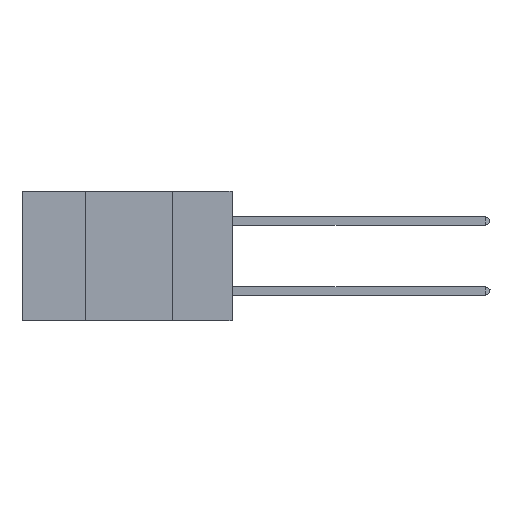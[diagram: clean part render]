
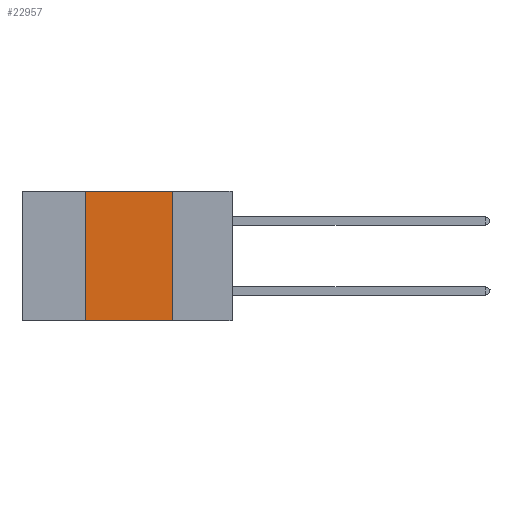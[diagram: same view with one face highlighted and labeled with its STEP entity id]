
A CAD part, left-side view. The second image highlights one B-rep face of the part: STEP entity #22957.
In plain terms, the highlighted planar face has unit normal (-1, 0, 0).
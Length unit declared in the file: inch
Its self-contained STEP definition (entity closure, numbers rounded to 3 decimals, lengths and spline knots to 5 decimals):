
#232 = LINE ( 'NONE', #357, #9091 ) ;
#357 = CARTESIAN_POINT ( 'NONE',  ( 0., 0.6, 0. ) ) ;
#1050 = FACE_OUTER_BOUND ( 'NONE', #24272, .T. ) ;
#2478 = CARTESIAN_POINT ( 'NONE',  ( 0., 0.17, 0. ) ) ;
#5051 = DIRECTION ( 'NONE',  ( 0., 0., 1. ) ) ;
#6407 = VERTEX_POINT ( 'NONE', #14930 ) ;
#6604 = CARTESIAN_POINT ( 'NONE',  ( 0., 0.6, -0.37 ) ) ;
#7446 = VECTOR ( 'NONE', #8625, 39.37008 ) ;
#7816 = EDGE_CURVE ( 'NONE', #10226, #15791, #10579, .T. ) ;
#7909 = CARTESIAN_POINT ( 'NONE',  ( 0., 0.17, -0.37 ) ) ;
#8434 = ORIENTED_EDGE ( 'NONE', *, *, #7816, .F. ) ;
#8625 = DIRECTION ( 'NONE',  ( 0., 0., -1. ) ) ;
#9072 = CARTESIAN_POINT ( 'NONE',  ( 0., 0.42, 0. ) ) ;
#9091 = VECTOR ( 'NONE', #21678, 39.37008 ) ;
#10021 = AXIS2_PLACEMENT_3D ( 'NONE', #11379, #24820, #11125 ) ;
#10226 = VERTEX_POINT ( 'NONE', #2478 ) ;
#10579 = LINE ( 'NONE', #18482, #7446 ) ;
#11125 = DIRECTION ( 'NONE',  ( 0., 0., -1. ) ) ;
#11379 = CARTESIAN_POINT ( 'NONE',  ( 0., 0.6, 0. ) ) ;
#13355 = VECTOR ( 'NONE', #22412, 39.37008 ) ;
#14791 = LINE ( 'NONE', #6604, #13355 ) ;
#14930 = CARTESIAN_POINT ( 'NONE',  ( 0., 0.42, 0. ) ) ;
#15285 = VECTOR ( 'NONE', #5051, 39.37008 ) ;
#15791 = VERTEX_POINT ( 'NONE', #7909 ) ;
#17333 = ORIENTED_EDGE ( 'NONE', *, *, #18242, .F. ) ;
#17668 = VERTEX_POINT ( 'NONE', #23040 ) ;
#18242 = EDGE_CURVE ( 'NONE', #6407, #10226, #232, .T. ) ;
#18482 = CARTESIAN_POINT ( 'NONE',  ( 0., 0.17, 0. ) ) ;
#20098 = EDGE_CURVE ( 'NONE', #17668, #6407, #22655, .T. ) ;
#21087 = PLANE ( 'NONE',  #10021 ) ;
#21678 = DIRECTION ( 'NONE',  ( 0., -1., 0. ) ) ;
#22412 = DIRECTION ( 'NONE',  ( 0., -1., 0. ) ) ;
#22655 = LINE ( 'NONE', #9072, #15285 ) ;
#22957 = ADVANCED_FACE ( 'NONE', ( #1050 ), #21087, .F. ) ;
#22970 = ORIENTED_EDGE ( 'NONE', *, *, #20098, .F. ) ;
#23040 = CARTESIAN_POINT ( 'NONE',  ( 0., 0.42, -0.37 ) ) ;
#24272 = EDGE_LOOP ( 'NONE', ( #8434, #17333, #22970, #24567 ) ) ;
#24341 = EDGE_CURVE ( 'NONE', #17668, #15791, #14791, .T. ) ;
#24567 = ORIENTED_EDGE ( 'NONE', *, *, #24341, .T. ) ;
#24820 = DIRECTION ( 'NONE',  ( 1., 0., 0. ) ) ;
